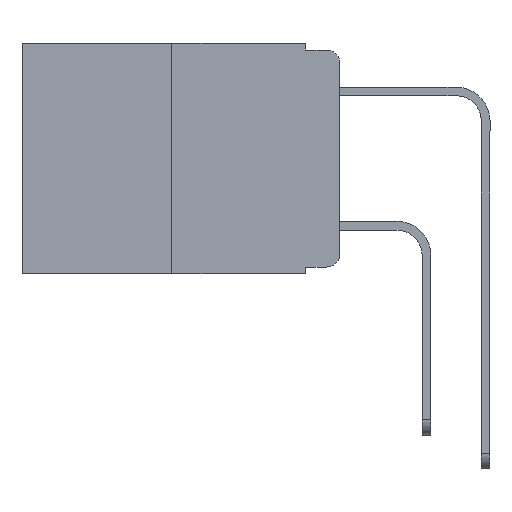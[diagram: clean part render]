
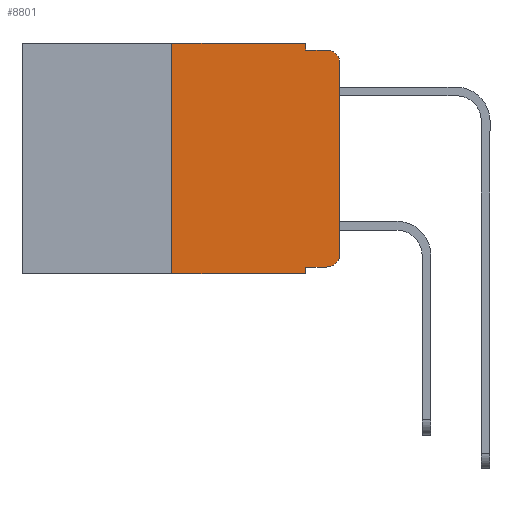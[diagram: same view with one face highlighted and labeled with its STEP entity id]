
A CAD part, left-side view. The second image highlights one B-rep face of the part: STEP entity #8801.
In plain terms, the highlighted planar face has unit normal (-1, 0, 0).
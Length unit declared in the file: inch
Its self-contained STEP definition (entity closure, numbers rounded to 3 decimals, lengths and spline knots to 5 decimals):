
#12 = FACE_OUTER_BOUND ( 'NONE', #10642, .T. ) ;
#332 = EDGE_CURVE ( 'NONE', #8526, #7896, #5432, .T. ) ;
#336 = CARTESIAN_POINT ( 'NONE',  ( 0., 0.051, -0.01 ) ) ;
#590 = EDGE_CURVE ( 'NONE', #12363, #12028, #4758, .T. ) ;
#616 = VECTOR ( 'NONE', #11872, 39.37008 ) ;
#692 = DIRECTION ( 'NONE',  ( 0., -1., 0. ) ) ;
#697 = DIRECTION ( 'NONE',  ( -1., 0., 0. ) ) ;
#949 = VERTEX_POINT ( 'NONE', #13032 ) ;
#1436 = CIRCLE ( 'NONE', #5878, 0.02 ) ;
#1474 = CARTESIAN_POINT ( 'NONE',  ( 0., 0.051, 0. ) ) ;
#1564 = CARTESIAN_POINT ( 'NONE',  ( 0., 0.02, -0.03 ) ) ;
#1600 = LINE ( 'NONE', #6315, #6890 ) ;
#1753 = ORIENTED_EDGE ( 'NONE', *, *, #8990, .F. ) ;
#1933 = CARTESIAN_POINT ( 'NONE',  ( 0., 0., -0.03 ) ) ;
#2111 = DIRECTION ( 'NONE',  ( 0., 0., 1. ) ) ;
#2141 = CARTESIAN_POINT ( 'NONE',  ( 0., 0.051, -0.333 ) ) ;
#2320 = VECTOR ( 'NONE', #692, 39.37008 ) ;
#2363 = CARTESIAN_POINT ( 'NONE',  ( 0., 0.051, 0. ) ) ;
#2508 = EDGE_CURVE ( 'NONE', #949, #12886, #11770, .T. ) ;
#2614 = DIRECTION ( 'NONE',  ( 0., 0., -1. ) ) ;
#2674 = EDGE_CURVE ( 'NONE', #12028, #4821, #1436, .T. ) ;
#2971 = VECTOR ( 'NONE', #8682, 39.37008 ) ;
#3050 = CARTESIAN_POINT ( 'NONE',  ( 0., 0.473, 0. ) ) ;
#3079 = ORIENTED_EDGE ( 'NONE', *, *, #590, .T. ) ;
#3191 = DIRECTION ( 'NONE',  ( 0., -1., 0. ) ) ;
#3511 = VERTEX_POINT ( 'NONE', #6295 ) ;
#3526 = EDGE_CURVE ( 'NONE', #3511, #8526, #4565, .T. ) ;
#3531 = VECTOR ( 'NONE', #11944, 39.37008 ) ;
#3831 = VECTOR ( 'NONE', #3191, 39.37008 ) ;
#4180 = EDGE_CURVE ( 'NONE', #4821, #11580, #1600, .T. ) ;
#4239 = ORIENTED_EDGE ( 'NONE', *, *, #3526, .F. ) ;
#4470 = LINE ( 'NONE', #10576, #3831 ) ;
#4565 = LINE ( 'NONE', #13529, #7081 ) ;
#4594 = ORIENTED_EDGE ( 'NONE', *, *, #332, .F. ) ;
#4758 = LINE ( 'NONE', #2141, #2320 ) ;
#4821 = VERTEX_POINT ( 'NONE', #11531 ) ;
#4933 = CARTESIAN_POINT ( 'NONE',  ( 0., 0.051, -0.343 ) ) ;
#4988 = ORIENTED_EDGE ( 'NONE', *, *, #2674, .T. ) ;
#5137 = DIRECTION ( 'NONE',  ( 0., -1., 0. ) ) ;
#5432 = LINE ( 'NONE', #8697, #8245 ) ;
#5653 = CARTESIAN_POINT ( 'NONE',  ( 0., 0.02, -0.01 ) ) ;
#5878 = AXIS2_PLACEMENT_3D ( 'NONE', #7012, #697, #8067 ) ;
#6240 = EDGE_CURVE ( 'NONE', #7896, #949, #11877, .T. ) ;
#6295 = CARTESIAN_POINT ( 'NONE',  ( 0., 0.25, -0.343 ) ) ;
#6315 = CARTESIAN_POINT ( 'NONE',  ( 0., 0., 0. ) ) ;
#6491 = VERTEX_POINT ( 'NONE', #4933 ) ;
#6689 = ORIENTED_EDGE ( 'NONE', *, *, #6240, .F. ) ;
#6890 = VECTOR ( 'NONE', #2111, 39.37008 ) ;
#7012 = CARTESIAN_POINT ( 'NONE',  ( 0., 0.02, -0.313 ) ) ;
#7081 = VECTOR ( 'NONE', #8409, 39.37008 ) ;
#7105 = CARTESIAN_POINT ( 'NONE',  ( 0., 0.02, -0.333 ) ) ;
#7139 = EDGE_CURVE ( 'NONE', #3511, #6491, #4470, .T. ) ;
#7314 = DIRECTION ( 'NONE',  ( 0., 0., -1. ) ) ;
#7329 = ORIENTED_EDGE ( 'NONE', *, *, #10105, .T. ) ;
#7412 = ORIENTED_EDGE ( 'NONE', *, *, #4180, .T. ) ;
#7896 = VERTEX_POINT ( 'NONE', #1474 ) ;
#7975 = CARTESIAN_POINT ( 'NONE',  ( 0., 0.051, -0.333 ) ) ;
#8037 = ORIENTED_EDGE ( 'NONE', *, *, #7139, .T. ) ;
#8067 = DIRECTION ( 'NONE',  ( 0., 0., -1. ) ) ;
#8245 = VECTOR ( 'NONE', #5137, 39.37008 ) ;
#8278 = AXIS2_PLACEMENT_3D ( 'NONE', #1564, #8935, #2614 ) ;
#8409 = DIRECTION ( 'NONE',  ( 0., 0., 1. ) ) ;
#8483 = CIRCLE ( 'NONE', #8278, 0.02 ) ;
#8526 = VERTEX_POINT ( 'NONE', #11975 ) ;
#8682 = DIRECTION ( 'NONE',  ( 0., 0., -1. ) ) ;
#8697 = CARTESIAN_POINT ( 'NONE',  ( 0., 0.473, 0. ) ) ;
#8801 = ADVANCED_FACE ( 'NONE', ( #12 ), #10399, .F. ) ;
#8935 = DIRECTION ( 'NONE',  ( -1., 0., 0. ) ) ;
#8990 = EDGE_CURVE ( 'NONE', #12363, #6491, #11335, .T. ) ;
#10105 = EDGE_CURVE ( 'NONE', #11580, #12886, #8483, .T. ) ;
#10142 = ORIENTED_EDGE ( 'NONE', *, *, #2508, .F. ) ;
#10399 = PLANE ( 'NONE',  #11456 ) ;
#10576 = CARTESIAN_POINT ( 'NONE',  ( 0., 0.473, -0.343 ) ) ;
#10642 = EDGE_LOOP ( 'NONE', ( #7412, #7329, #10142, #6689, #4594, #4239, #8037, #1753, #3079, #4988 ) ) ;
#10922 = CARTESIAN_POINT ( 'NONE',  ( 0., 0.051, 0. ) ) ;
#11335 = LINE ( 'NONE', #2363, #2971 ) ;
#11456 = AXIS2_PLACEMENT_3D ( 'NONE', #3050, #13480, #7314 ) ;
#11531 = CARTESIAN_POINT ( 'NONE',  ( 0., 0., -0.313 ) ) ;
#11580 = VERTEX_POINT ( 'NONE', #1933 ) ;
#11770 = LINE ( 'NONE', #336, #616 ) ;
#11872 = DIRECTION ( 'NONE',  ( 0., -1., 0. ) ) ;
#11877 = LINE ( 'NONE', #10922, #3531 ) ;
#11944 = DIRECTION ( 'NONE',  ( 0., 0., -1. ) ) ;
#11975 = CARTESIAN_POINT ( 'NONE',  ( 0., 0.25, 0. ) ) ;
#12028 = VERTEX_POINT ( 'NONE', #7105 ) ;
#12363 = VERTEX_POINT ( 'NONE', #7975 ) ;
#12886 = VERTEX_POINT ( 'NONE', #5653 ) ;
#13032 = CARTESIAN_POINT ( 'NONE',  ( 0., 0.051, -0.01 ) ) ;
#13480 = DIRECTION ( 'NONE',  ( 1., 0., 0. ) ) ;
#13529 = CARTESIAN_POINT ( 'NONE',  ( 0., 0.25, 0. ) ) ;
